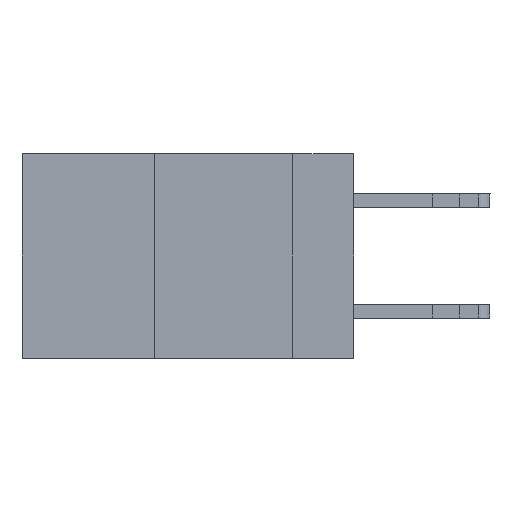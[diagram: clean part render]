
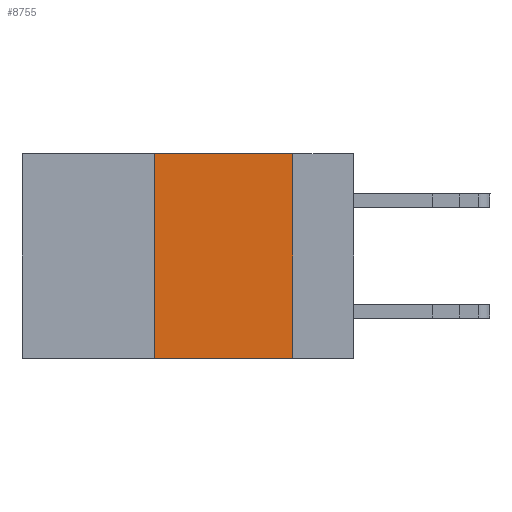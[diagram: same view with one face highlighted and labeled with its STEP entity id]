
A CAD part, left-side view. The second image highlights one B-rep face of the part: STEP entity #8755.
In plain terms, the highlighted planar face has unit normal (-1, 0, 0).
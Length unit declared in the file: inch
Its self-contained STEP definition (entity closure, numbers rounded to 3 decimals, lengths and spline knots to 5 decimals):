
#138 = LINE ( 'NONE', #3537, #11047 ) ;
#1244 = VECTOR ( 'NONE', #20454, 39.37008 ) ;
#1388 = LINE ( 'NONE', #17805, #1244 ) ;
#3537 = CARTESIAN_POINT ( 'NONE',  ( 0., 0.6, 0. ) ) ;
#3739 = DIRECTION ( 'NONE',  ( 0., -1., 0. ) ) ;
#3854 = VERTEX_POINT ( 'NONE', #22581 ) ;
#4034 = LINE ( 'NONE', #15890, #19439 ) ;
#7554 = CARTESIAN_POINT ( 'NONE',  ( 0., 0.11, 0. ) ) ;
#8029 = DIRECTION ( 'NONE',  ( 0., 0., -1. ) ) ;
#8755 = ADVANCED_FACE ( 'NONE', ( #22100 ), #19300, .F. ) ;
#10361 = EDGE_CURVE ( 'NONE', #21532, #15254, #27054, .T. ) ;
#11047 = VECTOR ( 'NONE', #21545, 39.37008 ) ;
#11279 = EDGE_CURVE ( 'NONE', #21224, #21532, #138, .T. ) ;
#12576 = DIRECTION ( 'NONE',  ( 0., 0., -1. ) ) ;
#12725 = CARTESIAN_POINT ( 'NONE',  ( 0., 0.11, 0. ) ) ;
#13386 = CARTESIAN_POINT ( 'NONE',  ( 0., 0.11, -0.37 ) ) ;
#15080 = CARTESIAN_POINT ( 'NONE',  ( 0., 0.6, 0. ) ) ;
#15213 = ORIENTED_EDGE ( 'NONE', *, *, #10361, .F. ) ;
#15254 = VERTEX_POINT ( 'NONE', #13386 ) ;
#15715 = AXIS2_PLACEMENT_3D ( 'NONE', #15080, #26775, #12576 ) ;
#15890 = CARTESIAN_POINT ( 'NONE',  ( 0., 0.6, -0.37 ) ) ;
#17805 = CARTESIAN_POINT ( 'NONE',  ( 0., 0.36, 0. ) ) ;
#18830 = CARTESIAN_POINT ( 'NONE',  ( 0., 0.36, 0. ) ) ;
#19300 = PLANE ( 'NONE',  #15715 ) ;
#19439 = VECTOR ( 'NONE', #3739, 39.37008 ) ;
#19982 = EDGE_LOOP ( 'NONE', ( #15213, #22665, #28035, #24046 ) ) ;
#20454 = DIRECTION ( 'NONE',  ( 0., 0., 1. ) ) ;
#21224 = VERTEX_POINT ( 'NONE', #18830 ) ;
#21532 = VERTEX_POINT ( 'NONE', #12725 ) ;
#21545 = DIRECTION ( 'NONE',  ( 0., -1., 0. ) ) ;
#21942 = EDGE_CURVE ( 'NONE', #3854, #21224, #1388, .T. ) ;
#22100 = FACE_OUTER_BOUND ( 'NONE', #19982, .T. ) ;
#22581 = CARTESIAN_POINT ( 'NONE',  ( 0., 0.36, -0.37 ) ) ;
#22665 = ORIENTED_EDGE ( 'NONE', *, *, #11279, .F. ) ;
#24046 = ORIENTED_EDGE ( 'NONE', *, *, #26929, .T. ) ;
#26775 = DIRECTION ( 'NONE',  ( 1., 0., 0. ) ) ;
#26929 = EDGE_CURVE ( 'NONE', #3854, #15254, #4034, .T. ) ;
#27054 = LINE ( 'NONE', #7554, #27745 ) ;
#27745 = VECTOR ( 'NONE', #8029, 39.37008 ) ;
#28035 = ORIENTED_EDGE ( 'NONE', *, *, #21942, .F. ) ;
